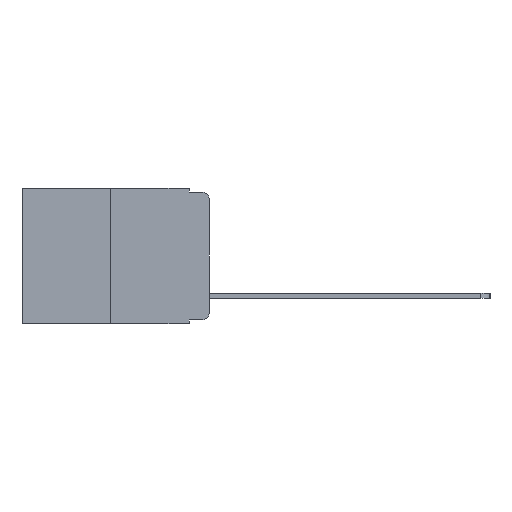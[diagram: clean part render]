
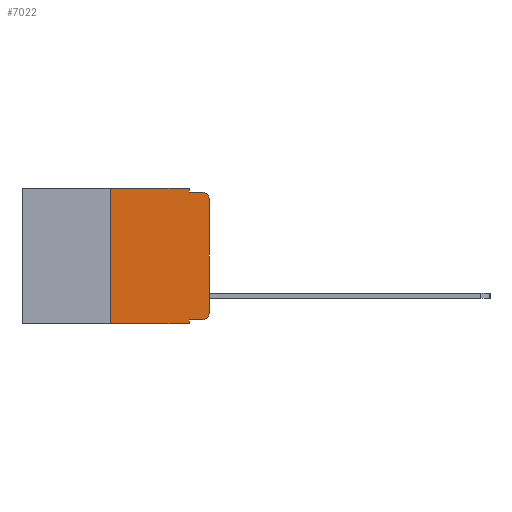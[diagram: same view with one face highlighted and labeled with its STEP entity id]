
A CAD part, left-side view. The second image highlights one B-rep face of the part: STEP entity #7022.
In plain terms, the highlighted planar face has unit normal (-1, 0, 0).
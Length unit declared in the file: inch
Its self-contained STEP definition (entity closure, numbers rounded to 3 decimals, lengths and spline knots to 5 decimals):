
#576 = CARTESIAN_POINT ( 'NONE',  ( 0., 0., -0.03 ) ) ;
#667 = EDGE_CURVE ( 'NONE', #19032, #11311, #19607, .T. ) ;
#1041 = DIRECTION ( 'NONE',  ( -1., 0., 0. ) ) ;
#1081 = LINE ( 'NONE', #11474, #5326 ) ;
#1133 = CIRCLE ( 'NONE', #10274, 0.02 ) ;
#1162 = CARTESIAN_POINT ( 'NONE',  ( 0., 0.02, -0.333 ) ) ;
#1201 = DIRECTION ( 'NONE',  ( 1., 0., 0. ) ) ;
#1453 = VECTOR ( 'NONE', #9149, 39.37008 ) ;
#1848 = VERTEX_POINT ( 'NONE', #2379 ) ;
#2033 = CARTESIAN_POINT ( 'NONE',  ( 0., 0.051, -0.343 ) ) ;
#2296 = DIRECTION ( 'NONE',  ( 0., 0., -1. ) ) ;
#2379 = CARTESIAN_POINT ( 'NONE',  ( 0., 0.02, -0.01 ) ) ;
#2443 = ORIENTED_EDGE ( 'NONE', *, *, #667, .T. ) ;
#2698 = EDGE_LOOP ( 'NONE', ( #3229, #2734, #11700, #6035, #10686, #15023, #2443, #14543, #3369, #15950 ) ) ;
#2734 = ORIENTED_EDGE ( 'NONE', *, *, #9231, .T. ) ;
#2913 = CARTESIAN_POINT ( 'NONE',  ( 0., 0.473, 0. ) ) ;
#3229 = ORIENTED_EDGE ( 'NONE', *, *, #16555, .T. ) ;
#3369 = ORIENTED_EDGE ( 'NONE', *, *, #5919, .T. ) ;
#3888 = DIRECTION ( 'NONE',  ( 0., 0., -1. ) ) ;
#3897 = LINE ( 'NONE', #19998, #20035 ) ;
#5326 = VECTOR ( 'NONE', #19140, 39.37008 ) ;
#5568 = DIRECTION ( 'NONE',  ( 0., 0., 1. ) ) ;
#5653 = CARTESIAN_POINT ( 'NONE',  ( 0., 0.25, 0. ) ) ;
#5919 = EDGE_CURVE ( 'NONE', #12545, #11634, #3897, .T. ) ;
#6035 = ORIENTED_EDGE ( 'NONE', *, *, #18484, .F. ) ;
#6198 = LINE ( 'NONE', #15386, #1453 ) ;
#6366 = VERTEX_POINT ( 'NONE', #11564 ) ;
#7022 = ADVANCED_FACE ( 'NONE', ( #11574 ), #12296, .F. ) ;
#7101 = DIRECTION ( 'NONE',  ( 0., -1., 0. ) ) ;
#7142 = EDGE_CURVE ( 'NONE', #11634, #6366, #1133, .T. ) ;
#7531 = AXIS2_PLACEMENT_3D ( 'NONE', #10540, #1041, #15783 ) ;
#8187 = EDGE_CURVE ( 'NONE', #19032, #20076, #19939, .T. ) ;
#9143 = VECTOR ( 'NONE', #11747, 39.37008 ) ;
#9149 = DIRECTION ( 'NONE',  ( 0., 0., -1. ) ) ;
#9231 = EDGE_CURVE ( 'NONE', #19974, #1848, #17372, .T. ) ;
#9305 = CARTESIAN_POINT ( 'NONE',  ( 0., 0.473, -0.343 ) ) ;
#9401 = VECTOR ( 'NONE', #14042, 39.37008 ) ;
#9610 = CARTESIAN_POINT ( 'NONE',  ( 0., 0., 0. ) ) ;
#10123 = CARTESIAN_POINT ( 'NONE',  ( 0., 0.473, 0. ) ) ;
#10190 = DIRECTION ( 'NONE',  ( -1., 0., 0. ) ) ;
#10206 = LINE ( 'NONE', #9610, #14385 ) ;
#10274 = AXIS2_PLACEMENT_3D ( 'NONE', #19459, #10190, #3888 ) ;
#10540 = CARTESIAN_POINT ( 'NONE',  ( 0., 0.02, -0.03 ) ) ;
#10580 = CARTESIAN_POINT ( 'NONE',  ( 0., 0.25, -0.343 ) ) ;
#10686 = ORIENTED_EDGE ( 'NONE', *, *, #18260, .F. ) ;
#10840 = VERTEX_POINT ( 'NONE', #18191 ) ;
#11311 = VERTEX_POINT ( 'NONE', #2033 ) ;
#11474 = CARTESIAN_POINT ( 'NONE',  ( 0., 0.051, -0.01 ) ) ;
#11564 = CARTESIAN_POINT ( 'NONE',  ( 0., 0., -0.313 ) ) ;
#11574 = FACE_OUTER_BOUND ( 'NONE', #2698, .T. ) ;
#11634 = VERTEX_POINT ( 'NONE', #1162 ) ;
#11700 = ORIENTED_EDGE ( 'NONE', *, *, #15527, .F. ) ;
#11747 = DIRECTION ( 'NONE',  ( 0., -1., 0. ) ) ;
#12296 = PLANE ( 'NONE',  #17929 ) ;
#12501 = CARTESIAN_POINT ( 'NONE',  ( 0., 0.051, 0. ) ) ;
#12545 = VERTEX_POINT ( 'NONE', #20077 ) ;
#13808 = LINE ( 'NONE', #10123, #9143 ) ;
#14042 = DIRECTION ( 'NONE',  ( 0., 0., -1. ) ) ;
#14289 = VERTEX_POINT ( 'NONE', #18465 ) ;
#14385 = VECTOR ( 'NONE', #18900, 39.37008 ) ;
#14415 = CARTESIAN_POINT ( 'NONE',  ( 0., 0.25, 0. ) ) ;
#14543 = ORIENTED_EDGE ( 'NONE', *, *, #17996, .F. ) ;
#14584 = VECTOR ( 'NONE', #16179, 39.37008 ) ;
#15023 = ORIENTED_EDGE ( 'NONE', *, *, #8187, .F. ) ;
#15386 = CARTESIAN_POINT ( 'NONE',  ( 0., 0.051, 0. ) ) ;
#15410 = VECTOR ( 'NONE', #5568, 39.37008 ) ;
#15527 = EDGE_CURVE ( 'NONE', #14289, #1848, #1081, .T. ) ;
#15783 = DIRECTION ( 'NONE',  ( 0., 0., -1. ) ) ;
#15950 = ORIENTED_EDGE ( 'NONE', *, *, #7142, .T. ) ;
#16179 = DIRECTION ( 'NONE',  ( 0., -1., 0. ) ) ;
#16555 = EDGE_CURVE ( 'NONE', #6366, #19974, #10206, .T. ) ;
#17372 = CIRCLE ( 'NONE', #7531, 0.02 ) ;
#17655 = LINE ( 'NONE', #12501, #9401 ) ;
#17929 = AXIS2_PLACEMENT_3D ( 'NONE', #2913, #1201, #2296 ) ;
#17996 = EDGE_CURVE ( 'NONE', #12545, #11311, #17655, .T. ) ;
#18191 = CARTESIAN_POINT ( 'NONE',  ( 0., 0.051, 0. ) ) ;
#18260 = EDGE_CURVE ( 'NONE', #20076, #10840, #13808, .T. ) ;
#18465 = CARTESIAN_POINT ( 'NONE',  ( 0., 0.051, -0.01 ) ) ;
#18484 = EDGE_CURVE ( 'NONE', #10840, #14289, #6198, .T. ) ;
#18900 = DIRECTION ( 'NONE',  ( 0., 0., 1. ) ) ;
#19032 = VERTEX_POINT ( 'NONE', #10580 ) ;
#19140 = DIRECTION ( 'NONE',  ( 0., -1., 0. ) ) ;
#19459 = CARTESIAN_POINT ( 'NONE',  ( 0., 0.02, -0.313 ) ) ;
#19607 = LINE ( 'NONE', #9305, #14584 ) ;
#19939 = LINE ( 'NONE', #14415, #15410 ) ;
#19974 = VERTEX_POINT ( 'NONE', #576 ) ;
#19998 = CARTESIAN_POINT ( 'NONE',  ( 0., 0.051, -0.333 ) ) ;
#20035 = VECTOR ( 'NONE', #7101, 39.37008 ) ;
#20076 = VERTEX_POINT ( 'NONE', #5653 ) ;
#20077 = CARTESIAN_POINT ( 'NONE',  ( 0., 0.051, -0.333 ) ) ;
